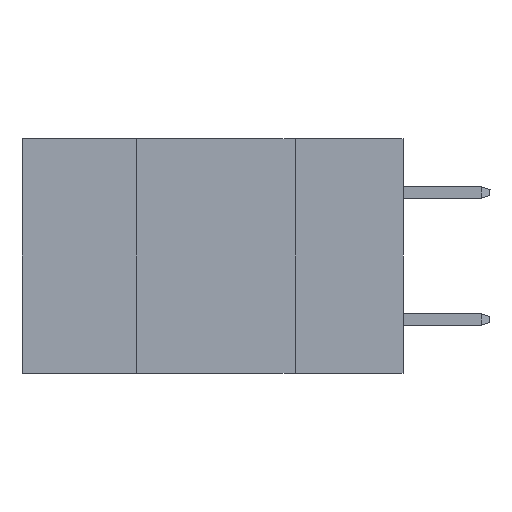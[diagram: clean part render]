
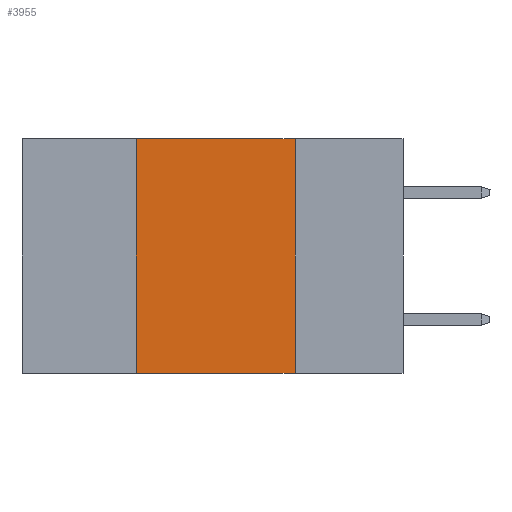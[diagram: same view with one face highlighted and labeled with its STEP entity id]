
A CAD part, left-side view. The second image highlights one B-rep face of the part: STEP entity #3955.
In plain terms, the highlighted planar face has unit normal (-1, 0, 0).
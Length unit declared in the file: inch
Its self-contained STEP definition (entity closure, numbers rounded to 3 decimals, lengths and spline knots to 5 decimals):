
#348 = DIRECTION ( 'NONE',  ( 0., 0., -1. ) ) ;
#739 = CARTESIAN_POINT ( 'NONE',  ( 0., 0.6, 0. ) ) ;
#827 = LINE ( 'NONE', #15146, #1961 ) ;
#1019 = LINE ( 'NONE', #739, #16065 ) ;
#1961 = VECTOR ( 'NONE', #7896, 39.37008 ) ;
#2699 = VERTEX_POINT ( 'NONE', #4380 ) ;
#3258 = LINE ( 'NONE', #16872, #10898 ) ;
#3955 = ADVANCED_FACE ( 'NONE', ( #15353 ), #18024, .F. ) ;
#4380 = CARTESIAN_POINT ( 'NONE',  ( 0., 0.42, 0. ) ) ;
#4387 = CARTESIAN_POINT ( 'NONE',  ( 0., 0.6, -0.37 ) ) ;
#4575 = VERTEX_POINT ( 'NONE', #17272 ) ;
#6123 = CARTESIAN_POINT ( 'NONE',  ( 0., 0.42, -0.37 ) ) ;
#6554 = VERTEX_POINT ( 'NONE', #17507 ) ;
#6692 = ORIENTED_EDGE ( 'NONE', *, *, #13024, .F. ) ;
#7061 = LINE ( 'NONE', #4387, #16366 ) ;
#7764 = EDGE_CURVE ( 'NONE', #13717, #2699, #827, .T. ) ;
#7896 = DIRECTION ( 'NONE',  ( 0., 0., 1. ) ) ;
#7958 = EDGE_CURVE ( 'NONE', #13717, #4575, #7061, .T. ) ;
#8360 = DIRECTION ( 'NONE',  ( 0., -1., 0. ) ) ;
#10251 = ORIENTED_EDGE ( 'NONE', *, *, #7958, .T. ) ;
#10375 = ORIENTED_EDGE ( 'NONE', *, *, #17811, .F. ) ;
#10898 = VECTOR ( 'NONE', #348, 39.37008 ) ;
#12067 = EDGE_LOOP ( 'NONE', ( #10375, #6692, #14559, #10251 ) ) ;
#13024 = EDGE_CURVE ( 'NONE', #2699, #6554, #1019, .T. ) ;
#13717 = VERTEX_POINT ( 'NONE', #6123 ) ;
#13722 = DIRECTION ( 'NONE',  ( 0., 0., -1. ) ) ;
#13871 = AXIS2_PLACEMENT_3D ( 'NONE', #15257, #17838, #13722 ) ;
#14559 = ORIENTED_EDGE ( 'NONE', *, *, #7764, .F. ) ;
#15146 = CARTESIAN_POINT ( 'NONE',  ( 0., 0.42, 0. ) ) ;
#15257 = CARTESIAN_POINT ( 'NONE',  ( 0., 0.6, 0. ) ) ;
#15353 = FACE_OUTER_BOUND ( 'NONE', #12067, .T. ) ;
#16065 = VECTOR ( 'NONE', #16332, 39.37008 ) ;
#16332 = DIRECTION ( 'NONE',  ( 0., -1., 0. ) ) ;
#16366 = VECTOR ( 'NONE', #8360, 39.37008 ) ;
#16872 = CARTESIAN_POINT ( 'NONE',  ( 0., 0.17, 0. ) ) ;
#17272 = CARTESIAN_POINT ( 'NONE',  ( 0., 0.17, -0.37 ) ) ;
#17507 = CARTESIAN_POINT ( 'NONE',  ( 0., 0.17, 0. ) ) ;
#17811 = EDGE_CURVE ( 'NONE', #6554, #4575, #3258, .T. ) ;
#17838 = DIRECTION ( 'NONE',  ( 1., 0., 0. ) ) ;
#18024 = PLANE ( 'NONE',  #13871 ) ;
